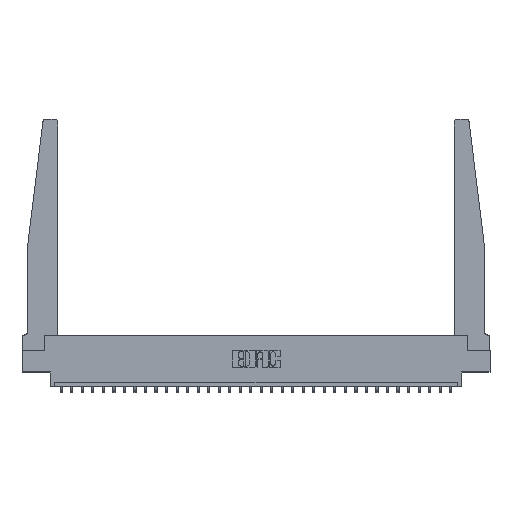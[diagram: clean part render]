
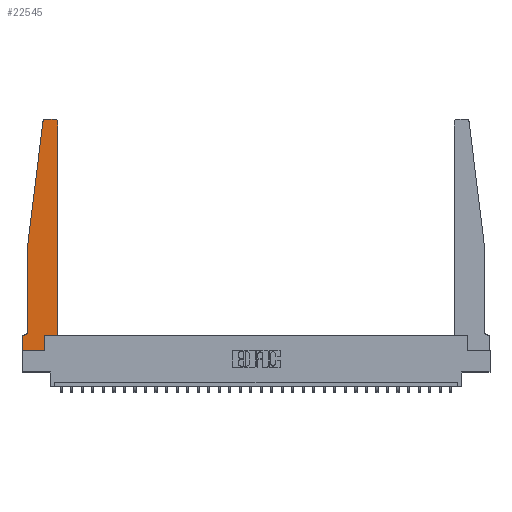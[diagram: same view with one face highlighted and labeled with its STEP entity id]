
A CAD part, top view. The second image highlights one B-rep face of the part: STEP entity #22545.
In plain terms, the highlighted planar face has unit normal (0, 0, 1).
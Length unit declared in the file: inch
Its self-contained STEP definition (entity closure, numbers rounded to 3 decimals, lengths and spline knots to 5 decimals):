
#288 = DIRECTION ( 'NONE',  ( -1., 0., 0. ) ) ;
#423 = VERTEX_POINT ( 'NONE', #8523 ) ;
#846 = ORIENTED_EDGE ( 'NONE', *, *, #27114, .T. ) ;
#1052 = LINE ( 'NONE', #10159, #22193 ) ;
#1089 = CARTESIAN_POINT ( 'NONE',  ( 0.425, 2.72, 0.37 ) ) ;
#1411 = ORIENTED_EDGE ( 'NONE', *, *, #11853, .T. ) ;
#1510 = DIRECTION ( 'NONE',  ( -1., 0., 0. ) ) ;
#2009 = DIRECTION ( 'NONE',  ( 1., 0., 0. ) ) ;
#3039 = LINE ( 'NONE', #12290, #20058 ) ;
#3068 = ORIENTED_EDGE ( 'NONE', *, *, #9184, .T. ) ;
#3454 = ORIENTED_EDGE ( 'NONE', *, *, #19073, .T. ) ;
#3606 = CARTESIAN_POINT ( 'NONE',  ( 0.015, 0.2375, 0.37 ) ) ;
#3810 = ORIENTED_EDGE ( 'NONE', *, *, #12286, .T. ) ;
#4281 = VERTEX_POINT ( 'NONE', #24576 ) ;
#4689 = CARTESIAN_POINT ( 'NONE',  ( 0.425, 0.18, 0.37 ) ) ;
#4848 = DIRECTION ( 'NONE',  ( 1., 0., 0. ) ) ;
#4861 = AXIS2_PLACEMENT_3D ( 'NONE', #14384, #14239, #23523 ) ;
#5103 = LINE ( 'NONE', #9288, #16240 ) ;
#5159 = DIRECTION ( 'NONE',  ( 0., -1., 0. ) ) ;
#5314 = CIRCLE ( 'NONE', #10090, 0.05 ) ;
#6206 = CARTESIAN_POINT ( 'NONE',  ( 0., 0., 0.37 ) ) ;
#6359 = VERTEX_POINT ( 'NONE', #8788 ) ;
#6437 = PLANE ( 'NONE',  #26119 ) ;
#6892 = DIRECTION ( 'NONE',  ( 1., 0., 0. ) ) ;
#6902 = DIRECTION ( 'NONE',  ( 0., -1., 0. ) ) ;
#6921 = EDGE_LOOP ( 'NONE', ( #17128, #9038, #3810, #3068, #9656, #9075, #28666, #9762, #3454, #23741, #1411, #846 ) ) ;
#7753 = VECTOR ( 'NONE', #5159, 39.37008 ) ;
#8375 = DIRECTION ( 'NONE',  ( 0., 0., -1. ) ) ;
#8523 = CARTESIAN_POINT ( 'NONE',  ( 0.065, 1.25, 0.37 ) ) ;
#8685 = FACE_OUTER_BOUND ( 'NONE', #6921, .T. ) ;
#8788 = CARTESIAN_POINT ( 'NONE',  ( 0.425, 0.18, 0.37 ) ) ;
#9038 = ORIENTED_EDGE ( 'NONE', *, *, #27276, .T. ) ;
#9075 = ORIENTED_EDGE ( 'NONE', *, *, #24651, .T. ) ;
#9178 = CARTESIAN_POINT ( 'NONE',  ( 0., 0., 0.37 ) ) ;
#9184 = EDGE_CURVE ( 'NONE', #423, #11720, #27452, .T. ) ;
#9288 = CARTESIAN_POINT ( 'NONE',  ( 0.065, 1.25, 0.37 ) ) ;
#9656 = ORIENTED_EDGE ( 'NONE', *, *, #28847, .T. ) ;
#9762 = ORIENTED_EDGE ( 'NONE', *, *, #20234, .T. ) ;
#9914 = VERTEX_POINT ( 'NONE', #20697 ) ;
#10090 = AXIS2_PLACEMENT_3D ( 'NONE', #3606, #8375, #1510 ) ;
#10159 = CARTESIAN_POINT ( 'NONE',  ( 0.2605, 0.18, 0.37 ) ) ;
#10234 = VERTEX_POINT ( 'NONE', #24287 ) ;
#10360 = CARTESIAN_POINT ( 'NONE',  ( 0.24675, 2.72367, 0.37 ) ) ;
#10781 = EDGE_CURVE ( 'NONE', #25322, #22046, #11374, .T. ) ;
#11223 = CARTESIAN_POINT ( 'NONE',  ( 0., 0., 0.37 ) ) ;
#11363 = CARTESIAN_POINT ( 'NONE',  ( 0.27653, 2.75, 0.37 ) ) ;
#11374 = LINE ( 'NONE', #11223, #19622 ) ;
#11547 = LINE ( 'NONE', #4689, #25493 ) ;
#11720 = VERTEX_POINT ( 'NONE', #22780 ) ;
#11853 = EDGE_CURVE ( 'NONE', #6359, #24029, #3039, .T. ) ;
#12143 = DIRECTION ( 'NONE',  ( 0., 1., 0. ) ) ;
#12286 = EDGE_CURVE ( 'NONE', #14388, #423, #5103, .T. ) ;
#12290 = CARTESIAN_POINT ( 'NONE',  ( 0.425, 0.18, 0.37 ) ) ;
#13305 = CARTESIAN_POINT ( 'NONE',  ( 0., 0.1875, 0.37 ) ) ;
#13641 = DIRECTION ( 'NONE',  ( 1., 0., 0. ) ) ;
#13823 = CARTESIAN_POINT ( 'NONE',  ( 0.395, 2.75, 0.37 ) ) ;
#14239 = DIRECTION ( 'NONE',  ( 0., 0., 1. ) ) ;
#14384 = CARTESIAN_POINT ( 'NONE',  ( 0.27653, 2.72, 0.37 ) ) ;
#14388 = VERTEX_POINT ( 'NONE', #10360 ) ;
#14693 = VECTOR ( 'NONE', #288, 39.37008 ) ;
#16240 = VECTOR ( 'NONE', #18957, 39.37008 ) ;
#16279 = AXIS2_PLACEMENT_3D ( 'NONE', #22477, #22783, #2009 ) ;
#16287 = VERTEX_POINT ( 'NONE', #11363 ) ;
#17128 = ORIENTED_EDGE ( 'NONE', *, *, #24318, .T. ) ;
#17148 = DIRECTION ( 'NONE',  ( 0., 1., 0. ) ) ;
#17552 = LINE ( 'NONE', #26714, #23827 ) ;
#17780 = EDGE_CURVE ( 'NONE', #10234, #6359, #11547, .T. ) ;
#18109 = LINE ( 'NONE', #9178, #29420 ) ;
#18763 = LINE ( 'NONE', #18909, #14693 ) ;
#18909 = CARTESIAN_POINT ( 'NONE',  ( 0.25, 2.75, 0.37 ) ) ;
#18957 = DIRECTION ( 'NONE',  ( -0.122, -0.992, 0. ) ) ;
#19073 = EDGE_CURVE ( 'NONE', #9914, #10234, #1052, .T. ) ;
#19622 = VECTOR ( 'NONE', #6902, 39.37008 ) ;
#19639 = CIRCLE ( 'NONE', #4861, 0.03 ) ;
#20058 = VECTOR ( 'NONE', #12143, 39.37008 ) ;
#20234 = EDGE_CURVE ( 'NONE', #22046, #9914, #18109, .T. ) ;
#20697 = CARTESIAN_POINT ( 'NONE',  ( 0.2605, 0., 0.37 ) ) ;
#22046 = VERTEX_POINT ( 'NONE', #6206 ) ;
#22193 = VECTOR ( 'NONE', #17148, 39.37008 ) ;
#22477 = CARTESIAN_POINT ( 'NONE',  ( 0.395, 2.72, 0.37 ) ) ;
#22545 = ADVANCED_FACE ( 'NONE', ( #8685 ), #6437, .T. ) ;
#22780 = CARTESIAN_POINT ( 'NONE',  ( 0.065, 0.2375, 0.37 ) ) ;
#22783 = DIRECTION ( 'NONE',  ( 0., 0., 1. ) ) ;
#22998 = CIRCLE ( 'NONE', #16279, 0.03 ) ;
#23501 = VERTEX_POINT ( 'NONE', #13823 ) ;
#23523 = DIRECTION ( 'NONE',  ( 1., 0., 0. ) ) ;
#23741 = ORIENTED_EDGE ( 'NONE', *, *, #17780, .T. ) ;
#23827 = VECTOR ( 'NONE', #29098, 39.37008 ) ;
#24029 = VERTEX_POINT ( 'NONE', #1089 ) ;
#24287 = CARTESIAN_POINT ( 'NONE',  ( 0.2605, 0.18, 0.37 ) ) ;
#24318 = EDGE_CURVE ( 'NONE', #23501, #16287, #18763, .T. ) ;
#24576 = CARTESIAN_POINT ( 'NONE',  ( 0.015, 0.1875, 0.37 ) ) ;
#24651 = EDGE_CURVE ( 'NONE', #4281, #25322, #17552, .T. ) ;
#25322 = VERTEX_POINT ( 'NONE', #28887 ) ;
#25493 = VECTOR ( 'NONE', #13641, 39.37008 ) ;
#25647 = CARTESIAN_POINT ( 'NONE',  ( 0.065, 1.25, 0.37 ) ) ;
#26119 = AXIS2_PLACEMENT_3D ( 'NONE', #13305, #29314, #6892 ) ;
#26714 = CARTESIAN_POINT ( 'NONE',  ( 0.065, 0.1875, 0.37 ) ) ;
#27114 = EDGE_CURVE ( 'NONE', #24029, #23501, #22998, .T. ) ;
#27276 = EDGE_CURVE ( 'NONE', #16287, #14388, #19639, .T. ) ;
#27452 = LINE ( 'NONE', #25647, #7753 ) ;
#28666 = ORIENTED_EDGE ( 'NONE', *, *, #10781, .T. ) ;
#28847 = EDGE_CURVE ( 'NONE', #11720, #4281, #5314, .T. ) ;
#28887 = CARTESIAN_POINT ( 'NONE',  ( 0., 0.1875, 0.37 ) ) ;
#29098 = DIRECTION ( 'NONE',  ( -1., 0., 0. ) ) ;
#29314 = DIRECTION ( 'NONE',  ( 0., 0., 1. ) ) ;
#29420 = VECTOR ( 'NONE', #4848, 39.37008 ) ;
